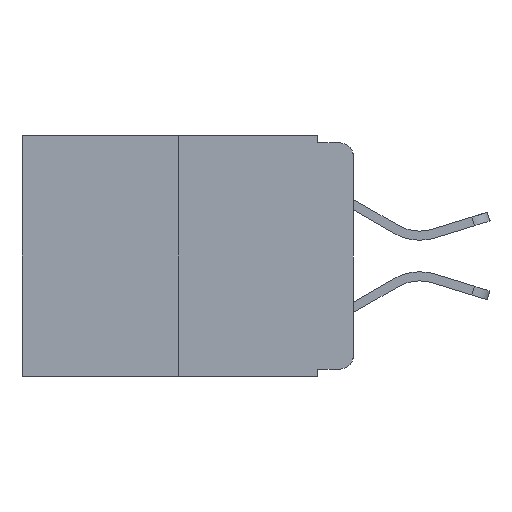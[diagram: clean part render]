
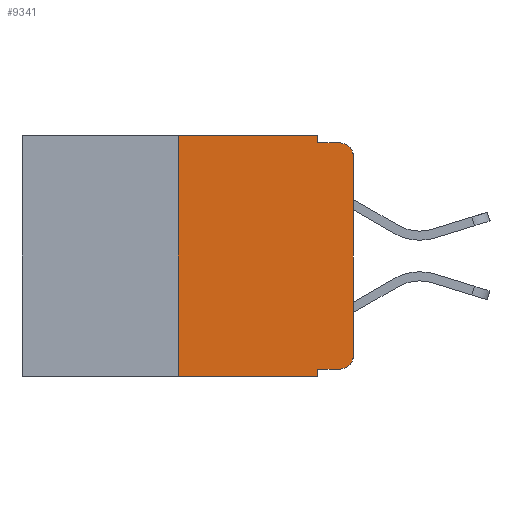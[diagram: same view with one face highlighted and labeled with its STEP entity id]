
A CAD part, left-side view. The second image highlights one B-rep face of the part: STEP entity #9341.
In plain terms, the highlighted planar face has unit normal (-1, 0, 0).
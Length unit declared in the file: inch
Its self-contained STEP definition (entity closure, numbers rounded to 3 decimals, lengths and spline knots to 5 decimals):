
#278 = VECTOR ( 'NONE', #10289, 39.37008 ) ;
#1392 = CARTESIAN_POINT ( 'NONE',  ( 0., 0.051, -0.333 ) ) ;
#1518 = VECTOR ( 'NONE', #7789, 39.37008 ) ;
#1606 = ORIENTED_EDGE ( 'NONE', *, *, #7762, .T. ) ;
#1684 = DIRECTION ( 'NONE',  ( 0., -1., 0. ) ) ;
#1714 = LINE ( 'NONE', #20852, #9517 ) ;
#1880 = EDGE_CURVE ( 'NONE', #22778, #8090, #6052, .T. ) ;
#2125 = CARTESIAN_POINT ( 'NONE',  ( 0., 0.25, 0. ) ) ;
#2863 = EDGE_CURVE ( 'NONE', #19205, #22223, #5020, .T. ) ;
#3064 = ORIENTED_EDGE ( 'NONE', *, *, #13209, .F. ) ;
#3290 = DIRECTION ( 'NONE',  ( 0., 0., -1. ) ) ;
#3322 = CARTESIAN_POINT ( 'NONE',  ( 0., 0.473, -0.343 ) ) ;
#3988 = EDGE_CURVE ( 'NONE', #14643, #13416, #18977, .T. ) ;
#4173 = ORIENTED_EDGE ( 'NONE', *, *, #7995, .T. ) ;
#4222 = CARTESIAN_POINT ( 'NONE',  ( 0., 0.051, -0.01 ) ) ;
#4261 = CARTESIAN_POINT ( 'NONE',  ( 0., 0.02, -0.03 ) ) ;
#4525 = CARTESIAN_POINT ( 'NONE',  ( 0., 0.02, -0.333 ) ) ;
#4644 = VERTEX_POINT ( 'NONE', #9856 ) ;
#4717 = VERTEX_POINT ( 'NONE', #1392 ) ;
#4838 = DIRECTION ( 'NONE',  ( 0., 0., -1. ) ) ;
#5020 = LINE ( 'NONE', #17701, #6155 ) ;
#5295 = VERTEX_POINT ( 'NONE', #4525 ) ;
#5804 = EDGE_CURVE ( 'NONE', #8090, #19205, #6943, .T. ) ;
#5857 = DIRECTION ( 'NONE',  ( -1., 0., 0. ) ) ;
#6052 = LINE ( 'NONE', #17074, #1518 ) ;
#6155 = VECTOR ( 'NONE', #1684, 39.37008 ) ;
#6492 = CARTESIAN_POINT ( 'NONE',  ( 0., 0.25, -0.343 ) ) ;
#6943 = LINE ( 'NONE', #17390, #22439 ) ;
#7762 = EDGE_CURVE ( 'NONE', #5295, #14643, #15750, .T. ) ;
#7782 = DIRECTION ( 'NONE',  ( 0., 0., 1. ) ) ;
#7789 = DIRECTION ( 'NONE',  ( 0., -1., 0. ) ) ;
#7857 = CARTESIAN_POINT ( 'NONE',  ( 0., 0., 0. ) ) ;
#7865 = ORIENTED_EDGE ( 'NONE', *, *, #5804, .F. ) ;
#7874 = ORIENTED_EDGE ( 'NONE', *, *, #3988, .T. ) ;
#7995 = EDGE_CURVE ( 'NONE', #4717, #5295, #15589, .T. ) ;
#8090 = VERTEX_POINT ( 'NONE', #20818 ) ;
#8277 = DIRECTION ( 'NONE',  ( 0., -1., 0. ) ) ;
#8281 = DIRECTION ( 'NONE',  ( 1., 0., 0. ) ) ;
#8787 = DIRECTION ( 'NONE',  ( 0., 0., -1. ) ) ;
#9341 = ADVANCED_FACE ( 'NONE', ( #22321 ), #13634, .F. ) ;
#9424 = LINE ( 'NONE', #2125, #22478 ) ;
#9517 = VECTOR ( 'NONE', #8787, 39.37008 ) ;
#9856 = CARTESIAN_POINT ( 'NONE',  ( 0., 0.051, -0.343 ) ) ;
#9885 = AXIS2_PLACEMENT_3D ( 'NONE', #4261, #18439, #22014 ) ;
#10040 = EDGE_CURVE ( 'NONE', #13416, #22223, #10246, .T. ) ;
#10207 = CARTESIAN_POINT ( 'NONE',  ( 0., 0., -0.313 ) ) ;
#10246 = CIRCLE ( 'NONE', #9885, 0.02 ) ;
#10289 = DIRECTION ( 'NONE',  ( 0., -1., 0. ) ) ;
#10971 = ORIENTED_EDGE ( 'NONE', *, *, #1880, .F. ) ;
#12213 = CARTESIAN_POINT ( 'NONE',  ( 0., 0.051, -0.333 ) ) ;
#13189 = EDGE_CURVE ( 'NONE', #16363, #4644, #15744, .T. ) ;
#13209 = EDGE_CURVE ( 'NONE', #4717, #4644, #1714, .T. ) ;
#13416 = VERTEX_POINT ( 'NONE', #16358 ) ;
#13634 = PLANE ( 'NONE',  #22821 ) ;
#14285 = CARTESIAN_POINT ( 'NONE',  ( 0., 0.25, 0. ) ) ;
#14643 = VERTEX_POINT ( 'NONE', #10207 ) ;
#14730 = DIRECTION ( 'NONE',  ( 0., 0., 1. ) ) ;
#15589 = LINE ( 'NONE', #12213, #22468 ) ;
#15707 = VECTOR ( 'NONE', #14730, 39.37008 ) ;
#15744 = LINE ( 'NONE', #3322, #278 ) ;
#15750 = CIRCLE ( 'NONE', #22391, 0.02 ) ;
#16358 = CARTESIAN_POINT ( 'NONE',  ( 0., 0., -0.03 ) ) ;
#16363 = VERTEX_POINT ( 'NONE', #6492 ) ;
#17074 = CARTESIAN_POINT ( 'NONE',  ( 0., 0.473, 0. ) ) ;
#17172 = ORIENTED_EDGE ( 'NONE', *, *, #13189, .T. ) ;
#17201 = CARTESIAN_POINT ( 'NONE',  ( 0., 0.02, -0.01 ) ) ;
#17224 = ORIENTED_EDGE ( 'NONE', *, *, #17739, .F. ) ;
#17390 = CARTESIAN_POINT ( 'NONE',  ( 0., 0.051, 0. ) ) ;
#17701 = CARTESIAN_POINT ( 'NONE',  ( 0., 0.051, -0.01 ) ) ;
#17739 = EDGE_CURVE ( 'NONE', #16363, #22778, #9424, .T. ) ;
#18439 = DIRECTION ( 'NONE',  ( -1., 0., 0. ) ) ;
#18594 = EDGE_LOOP ( 'NONE', ( #7874, #19898, #20510, #7865, #10971, #17224, #17172, #3064, #4173, #1606 ) ) ;
#18977 = LINE ( 'NONE', #7857, #15707 ) ;
#19205 = VERTEX_POINT ( 'NONE', #4222 ) ;
#19690 = DIRECTION ( 'NONE',  ( 0., 0., -1. ) ) ;
#19898 = ORIENTED_EDGE ( 'NONE', *, *, #10040, .T. ) ;
#20510 = ORIENTED_EDGE ( 'NONE', *, *, #2863, .F. ) ;
#20593 = CARTESIAN_POINT ( 'NONE',  ( 0., 0.473, 0. ) ) ;
#20818 = CARTESIAN_POINT ( 'NONE',  ( 0., 0.051, 0. ) ) ;
#20852 = CARTESIAN_POINT ( 'NONE',  ( 0., 0.051, 0. ) ) ;
#21648 = CARTESIAN_POINT ( 'NONE',  ( 0., 0.02, -0.313 ) ) ;
#22014 = DIRECTION ( 'NONE',  ( 0., 0., -1. ) ) ;
#22223 = VERTEX_POINT ( 'NONE', #17201 ) ;
#22321 = FACE_OUTER_BOUND ( 'NONE', #18594, .T. ) ;
#22391 = AXIS2_PLACEMENT_3D ( 'NONE', #21648, #5857, #19690 ) ;
#22439 = VECTOR ( 'NONE', #4838, 39.37008 ) ;
#22468 = VECTOR ( 'NONE', #8277, 39.37008 ) ;
#22478 = VECTOR ( 'NONE', #7782, 39.37008 ) ;
#22778 = VERTEX_POINT ( 'NONE', #14285 ) ;
#22821 = AXIS2_PLACEMENT_3D ( 'NONE', #20593, #8281, #3290 ) ;
